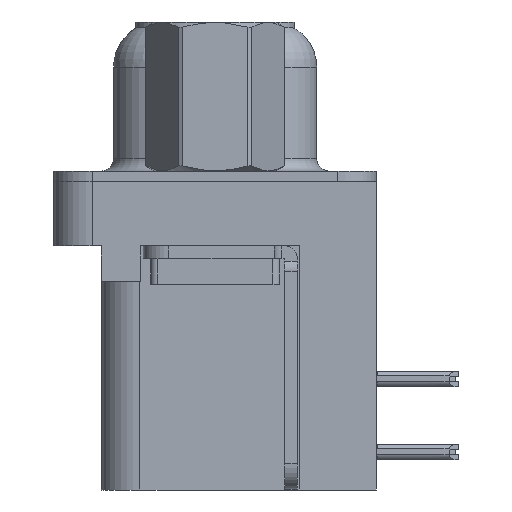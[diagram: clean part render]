
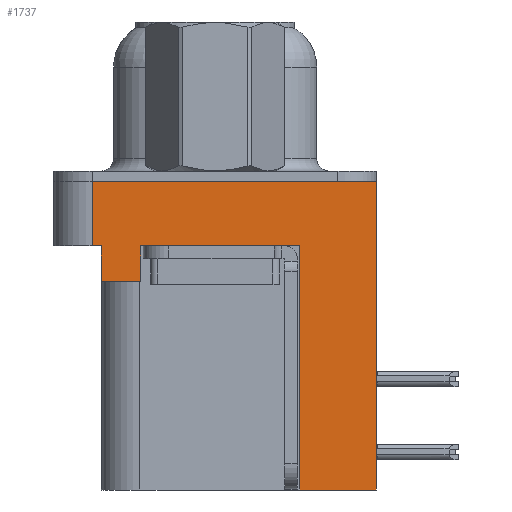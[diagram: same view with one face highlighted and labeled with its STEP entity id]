
A CAD part, left-side view. The second image highlights one B-rep face of the part: STEP entity #1737.
In plain terms, the highlighted planar face has unit normal (-1, 0, 0).
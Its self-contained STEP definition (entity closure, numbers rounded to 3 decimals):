
#136 = LINE ( 'NONE', #10650, #19442 ) ;
#653 = ORIENTED_EDGE ( 'NONE', *, *, #25957, .T. ) ;
#1003 = FACE_OUTER_BOUND ( 'NONE', #30436, .T. ) ;
#1703 = DIRECTION ( 'NONE',  ( -1., 0., 0. ) ) ;
#1737 = ADVANCED_FACE ( 'NONE', ( #1003 ), #3599, .T. ) ;
#2128 = CARTESIAN_POINT ( 'NONE',  ( -2.935, 4.775, 0. ) ) ;
#3599 = PLANE ( 'NONE',  #14956 ) ;
#3890 = VECTOR ( 'NONE', #26167, 1000. ) ;
#4565 = VECTOR ( 'NONE', #26297, 1000. ) ;
#4591 = ORIENTED_EDGE ( 'NONE', *, *, #5843, .F. ) ;
#4780 = CARTESIAN_POINT ( 'NONE',  ( -2.935, -6.275, -2.5 ) ) ;
#4965 = LINE ( 'NONE', #24761, #12011 ) ;
#5103 = LINE ( 'NONE', #25497, #6920 ) ;
#5636 = DIRECTION ( 'NONE',  ( 0., -1., 0. ) ) ;
#5802 = VERTEX_POINT ( 'NONE', #15036 ) ;
#5843 = EDGE_CURVE ( 'NONE', #26412, #8064, #10844, .T. ) ;
#6483 = VERTEX_POINT ( 'NONE', #27120 ) ;
#6590 = VECTOR ( 'NONE', #10315, 1000. ) ;
#6676 = VECTOR ( 'NONE', #6921, 1000. ) ;
#6920 = VECTOR ( 'NONE', #27918, 1000. ) ;
#6921 = DIRECTION ( 'NONE',  ( 0., 1., 0. ) ) ;
#8064 = VERTEX_POINT ( 'NONE', #24963 ) ;
#8586 = CARTESIAN_POINT ( 'NONE',  ( -2.935, -3.295, -2.5 ) ) ;
#9040 = VERTEX_POINT ( 'NONE', #8586 ) ;
#9245 = CARTESIAN_POINT ( 'NONE',  ( -2.935, -6.275, -2.5 ) ) ;
#9380 = LINE ( 'NONE', #27853, #14886 ) ;
#9695 = CARTESIAN_POINT ( 'NONE',  ( -2.935, 4.425, -3.9 ) ) ;
#9831 = LINE ( 'NONE', #4780, #3890 ) ;
#10315 = DIRECTION ( 'NONE',  ( 0., 0., 1. ) ) ;
#10650 = CARTESIAN_POINT ( 'NONE',  ( -2.935, -3.295, -12. ) ) ;
#10844 = LINE ( 'NONE', #9695, #4565 ) ;
#12011 = VECTOR ( 'NONE', #17271, 1000. ) ;
#13391 = ORIENTED_EDGE ( 'NONE', *, *, #25127, .F. ) ;
#13713 = CARTESIAN_POINT ( 'NONE',  ( -2.935, 2.895, -3.9 ) ) ;
#13748 = CARTESIAN_POINT ( 'NONE',  ( -2.935, -6.275, -12. ) ) ;
#14807 = LINE ( 'NONE', #28574, #6676 ) ;
#14886 = VECTOR ( 'NONE', #28286, 1000. ) ;
#14956 = AXIS2_PLACEMENT_3D ( 'NONE', #23317, #1703, #20811 ) ;
#15036 = CARTESIAN_POINT ( 'NONE',  ( -2.935, -6.275, 0. ) ) ;
#15418 = DIRECTION ( 'NONE',  ( 0., 0., 1. ) ) ;
#15715 = CARTESIAN_POINT ( 'NONE',  ( -2.935, 4.425, -2.5 ) ) ;
#15957 = ORIENTED_EDGE ( 'NONE', *, *, #24481, .F. ) ;
#16533 = ORIENTED_EDGE ( 'NONE', *, *, #19669, .T. ) ;
#17152 = VECTOR ( 'NONE', #25820, 1000. ) ;
#17271 = DIRECTION ( 'NONE',  ( 0., 0., 1. ) ) ;
#18083 = CARTESIAN_POINT ( 'NONE',  ( -2.935, -3.295, -12. ) ) ;
#18673 = EDGE_CURVE ( 'NONE', #28222, #9040, #9831, .T. ) ;
#18910 = ORIENTED_EDGE ( 'NONE', *, *, #18673, .T. ) ;
#19404 = CARTESIAN_POINT ( 'NONE',  ( -2.935, 2.895, -2.5 ) ) ;
#19415 = LINE ( 'NONE', #9245, #17152 ) ;
#19442 = VECTOR ( 'NONE', #15418, 1000. ) ;
#19568 = LINE ( 'NONE', #24625, #6590 ) ;
#19669 = EDGE_CURVE ( 'NONE', #23658, #5802, #19568, .T. ) ;
#20194 = VERTEX_POINT ( 'NONE', #18083 ) ;
#20754 = EDGE_CURVE ( 'NONE', #23658, #20194, #14807, .T. ) ;
#20811 = DIRECTION ( 'NONE',  ( 0., 0., 1. ) ) ;
#21128 = ORIENTED_EDGE ( 'NONE', *, *, #20754, .F. ) ;
#21288 = VECTOR ( 'NONE', #5636, 1000. ) ;
#23317 = CARTESIAN_POINT ( 'NONE',  ( -2.935, -6.275, -2.5 ) ) ;
#23658 = VERTEX_POINT ( 'NONE', #13748 ) ;
#24481 = EDGE_CURVE ( 'NONE', #6483, #27217, #4965, .T. ) ;
#24505 = ORIENTED_EDGE ( 'NONE', *, *, #28313, .F. ) ;
#24625 = CARTESIAN_POINT ( 'NONE',  ( -2.935, -6.275, -2.5 ) ) ;
#24636 = ORIENTED_EDGE ( 'NONE', *, *, #29687, .F. ) ;
#24761 = CARTESIAN_POINT ( 'NONE',  ( -2.935, 4.775, -2.5 ) ) ;
#24963 = CARTESIAN_POINT ( 'NONE',  ( -2.935, 4.425, -3.9 ) ) ;
#25127 = EDGE_CURVE ( 'NONE', #27217, #5802, #29139, .T. ) ;
#25497 = CARTESIAN_POINT ( 'NONE',  ( -2.935, 2.895, -3.9 ) ) ;
#25820 = DIRECTION ( 'NONE',  ( 0., -1., 0. ) ) ;
#25950 = VERTEX_POINT ( 'NONE', #15715 ) ;
#25957 = EDGE_CURVE ( 'NONE', #26412, #28222, #5103, .T. ) ;
#26167 = DIRECTION ( 'NONE',  ( 0., -1., 0. ) ) ;
#26297 = DIRECTION ( 'NONE',  ( 0., 1., 0. ) ) ;
#26412 = VERTEX_POINT ( 'NONE', #13713 ) ;
#27120 = CARTESIAN_POINT ( 'NONE',  ( -2.935, 4.775, -2.5 ) ) ;
#27217 = VERTEX_POINT ( 'NONE', #2128 ) ;
#27810 = ORIENTED_EDGE ( 'NONE', *, *, #29334, .T. ) ;
#27853 = CARTESIAN_POINT ( 'NONE',  ( -2.935, 4.425, -3.9 ) ) ;
#27918 = DIRECTION ( 'NONE',  ( 0., 0., 1. ) ) ;
#28222 = VERTEX_POINT ( 'NONE', #19404 ) ;
#28286 = DIRECTION ( 'NONE',  ( 0., 0., 1. ) ) ;
#28313 = EDGE_CURVE ( 'NONE', #20194, #9040, #136, .T. ) ;
#28574 = CARTESIAN_POINT ( 'NONE',  ( -2.935, -3.295, -12. ) ) ;
#29139 = LINE ( 'NONE', #29470, #21288 ) ;
#29334 = EDGE_CURVE ( 'NONE', #6483, #25950, #19415, .T. ) ;
#29470 = CARTESIAN_POINT ( 'NONE',  ( -2.935, -6.275, 0. ) ) ;
#29687 = EDGE_CURVE ( 'NONE', #8064, #25950, #9380, .T. ) ;
#30436 = EDGE_LOOP ( 'NONE', ( #13391, #15957, #27810, #24636, #4591, #653, #18910, #24505, #21128, #16533 ) ) ;
